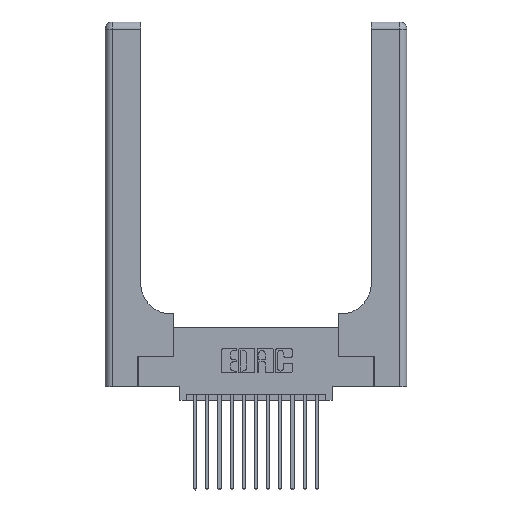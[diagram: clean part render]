
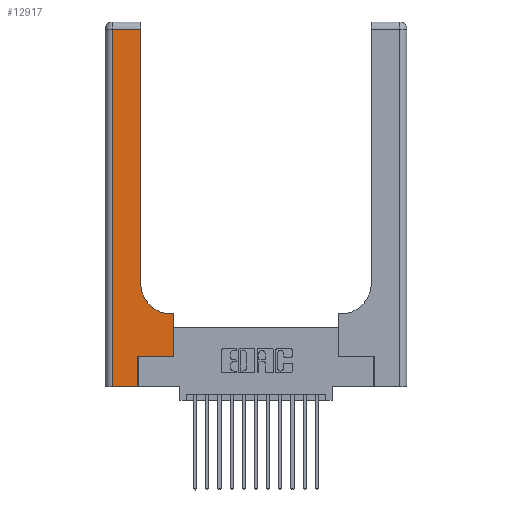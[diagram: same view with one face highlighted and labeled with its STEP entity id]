
A CAD part, top view. The second image highlights one B-rep face of the part: STEP entity #12917.
In plain terms, the highlighted planar face has unit normal (0, 0, 1).
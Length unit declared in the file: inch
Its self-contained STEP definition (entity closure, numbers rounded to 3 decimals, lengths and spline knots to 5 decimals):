
#30 = EDGE_CURVE ( 'NONE', #5347, #4898, #17592, .T. ) ;
#113 = DIRECTION ( 'NONE',  ( 0., 1., 0. ) ) ;
#523 = CARTESIAN_POINT ( 'NONE',  ( 0.5585, 0.25, 0.37 ) ) ;
#671 = DIRECTION ( 'NONE',  ( -1., 0., 0. ) ) ;
#1389 = DIRECTION ( 'NONE',  ( -1., 0., 0. ) ) ;
#1402 = VECTOR ( 'NONE', #12056, 39.37008 ) ;
#1689 = VERTEX_POINT ( 'NONE', #6189 ) ;
#1699 = VERTEX_POINT ( 'NONE', #9126 ) ;
#1834 = LINE ( 'NONE', #523, #1402 ) ;
#2170 = CARTESIAN_POINT ( 'NONE',  ( 0.269, 0.25, 0.37 ) ) ;
#2561 = CARTESIAN_POINT ( 'NONE',  ( 0.269, 0., 0.37 ) ) ;
#2674 = VECTOR ( 'NONE', #11940, 39.37008 ) ;
#2724 = ORIENTED_EDGE ( 'NONE', *, *, #6367, .T. ) ;
#2975 = ORIENTED_EDGE ( 'NONE', *, *, #11476, .T. ) ;
#3088 = LINE ( 'NONE', #2170, #6405 ) ;
#3493 = VECTOR ( 'NONE', #12031, 39.37008 ) ;
#3581 = VERTEX_POINT ( 'NONE', #6944 ) ;
#4202 = ORIENTED_EDGE ( 'NONE', *, *, #6622, .T. ) ;
#4307 = CARTESIAN_POINT ( 'NONE',  ( 0., 3., 0.37 ) ) ;
#4410 = VECTOR ( 'NONE', #4675, 39.37008 ) ;
#4605 = CARTESIAN_POINT ( 'NONE',  ( 0., 2.94, 0.37 ) ) ;
#4629 = LINE ( 'NONE', #17799, #2674 ) ;
#4650 = CIRCLE ( 'NONE', #16667, 0.25 ) ;
#4675 = DIRECTION ( 'NONE',  ( 0., 1., 0. ) ) ;
#4898 = VERTEX_POINT ( 'NONE', #17523 ) ;
#5089 = ORIENTED_EDGE ( 'NONE', *, *, #8305, .T. ) ;
#5347 = VERTEX_POINT ( 'NONE', #5803 ) ;
#5388 = ORIENTED_EDGE ( 'NONE', *, *, #15231, .T. ) ;
#5588 = CARTESIAN_POINT ( 'NONE',  ( 0.06, 0., 0.37 ) ) ;
#5803 = CARTESIAN_POINT ( 'NONE',  ( 0.269, 0., 0.37 ) ) ;
#6146 = LINE ( 'NONE', #10458, #14277 ) ;
#6150 = EDGE_CURVE ( 'NONE', #1689, #17697, #1834, .T. ) ;
#6189 = CARTESIAN_POINT ( 'NONE',  ( 0.5585, 0.25, 0.37 ) ) ;
#6367 = EDGE_CURVE ( 'NONE', #3581, #1699, #4650, .T. ) ;
#6405 = VECTOR ( 'NONE', #14704, 39.37008 ) ;
#6622 = EDGE_CURVE ( 'NONE', #1699, #9783, #16547, .T. ) ;
#6944 = CARTESIAN_POINT ( 'NONE',  ( 0.5415, 0.6, 0.37 ) ) ;
#7196 = ORIENTED_EDGE ( 'NONE', *, *, #10203, .T. ) ;
#8305 = EDGE_CURVE ( 'NONE', #12093, #5347, #17860, .T. ) ;
#8822 = DIRECTION ( 'NONE',  ( 1., 0., 0. ) ) ;
#9000 = EDGE_LOOP ( 'NONE', ( #4202, #2975, #5388, #5089, #13927, #7196, #17409, #14369, #2724 ) ) ;
#9126 = CARTESIAN_POINT ( 'NONE',  ( 0.2915, 0.85, 0.37 ) ) ;
#9180 = AXIS2_PLACEMENT_3D ( 'NONE', #4307, #9666, #1389 ) ;
#9356 = CARTESIAN_POINT ( 'NONE',  ( 0.06, 2.94, 0.37 ) ) ;
#9432 = LINE ( 'NONE', #4605, #3493 ) ;
#9479 = VECTOR ( 'NONE', #113, 39.37008 ) ;
#9482 = DIRECTION ( 'NONE',  ( 0., 0., -1. ) ) ;
#9666 = DIRECTION ( 'NONE',  ( 0., 0., -1. ) ) ;
#9783 = VERTEX_POINT ( 'NONE', #14131 ) ;
#9786 = PLANE ( 'NONE',  #9180 ) ;
#10203 = EDGE_CURVE ( 'NONE', #4898, #1689, #3088, .T. ) ;
#10458 = CARTESIAN_POINT ( 'NONE',  ( 0.2915, 0.6, 0.37 ) ) ;
#11065 = CARTESIAN_POINT ( 'NONE',  ( 0.5415, 0.85, 0.37 ) ) ;
#11234 = EDGE_CURVE ( 'NONE', #17697, #3581, #6146, .T. ) ;
#11316 = FACE_OUTER_BOUND ( 'NONE', #9000, .T. ) ;
#11476 = EDGE_CURVE ( 'NONE', #9783, #16490, #9432, .T. ) ;
#11940 = DIRECTION ( 'NONE',  ( 0., -1., 0. ) ) ;
#12031 = DIRECTION ( 'NONE',  ( -1., 0., 0. ) ) ;
#12056 = DIRECTION ( 'NONE',  ( 0., 1., 0. ) ) ;
#12093 = VERTEX_POINT ( 'NONE', #5588 ) ;
#12776 = VECTOR ( 'NONE', #8822, 39.37008 ) ;
#12917 = ADVANCED_FACE ( 'NONE', ( #11316 ), #9786, .F. ) ;
#13927 = ORIENTED_EDGE ( 'NONE', *, *, #30, .T. ) ;
#14131 = CARTESIAN_POINT ( 'NONE',  ( 0.2915, 2.94, 0.37 ) ) ;
#14277 = VECTOR ( 'NONE', #671, 39.37008 ) ;
#14369 = ORIENTED_EDGE ( 'NONE', *, *, #11234, .T. ) ;
#14704 = DIRECTION ( 'NONE',  ( 1., 0., 0. ) ) ;
#15046 = CARTESIAN_POINT ( 'NONE',  ( 0.5585, 0.6, 0.37 ) ) ;
#15231 = EDGE_CURVE ( 'NONE', #16490, #12093, #4629, .T. ) ;
#15997 = CARTESIAN_POINT ( 'NONE',  ( 0.2915, 3., 0.37 ) ) ;
#16490 = VERTEX_POINT ( 'NONE', #9356 ) ;
#16547 = LINE ( 'NONE', #15997, #4410 ) ;
#16572 = DIRECTION ( 'NONE',  ( 1., 0., 0. ) ) ;
#16667 = AXIS2_PLACEMENT_3D ( 'NONE', #11065, #9482, #16572 ) ;
#17242 = CARTESIAN_POINT ( 'NONE',  ( 0., 0., 0.37 ) ) ;
#17409 = ORIENTED_EDGE ( 'NONE', *, *, #6150, .T. ) ;
#17523 = CARTESIAN_POINT ( 'NONE',  ( 0.269, 0.25, 0.37 ) ) ;
#17592 = LINE ( 'NONE', #2561, #9479 ) ;
#17697 = VERTEX_POINT ( 'NONE', #15046 ) ;
#17799 = CARTESIAN_POINT ( 'NONE',  ( 0.06, 3., 0.37 ) ) ;
#17860 = LINE ( 'NONE', #17242, #12776 ) ;
